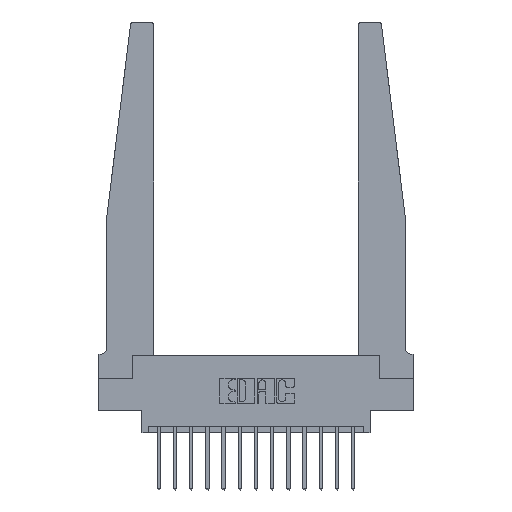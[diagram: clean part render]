
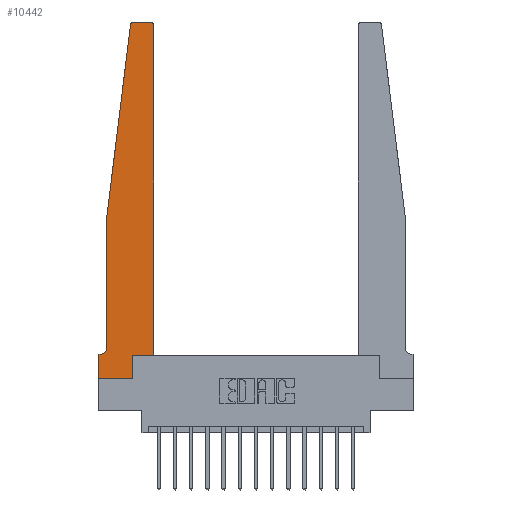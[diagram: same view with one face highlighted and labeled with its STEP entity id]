
A CAD part, top view. The second image highlights one B-rep face of the part: STEP entity #10442.
In plain terms, the highlighted planar face has unit normal (0, 0, 1).
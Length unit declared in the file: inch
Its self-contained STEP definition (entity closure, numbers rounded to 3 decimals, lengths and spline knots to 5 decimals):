
#40 = CARTESIAN_POINT ( 'NONE',  ( 0.395, 2.72, 0.37 ) ) ;
#259 = DIRECTION ( 'NONE',  ( 0., 1., 0. ) ) ;
#263 = AXIS2_PLACEMENT_3D ( 'NONE', #17476, #5307, #6751 ) ;
#320 = VECTOR ( 'NONE', #13729, 39.37008 ) ;
#450 = CARTESIAN_POINT ( 'NONE',  ( 0.015, 0.2375, 0.37 ) ) ;
#515 = LINE ( 'NONE', #7627, #7411 ) ;
#552 = EDGE_LOOP ( 'NONE', ( #8820, #11416, #11705, #750, #2528, #7859, #1773, #2253, #5050, #16981, #3275, #9507 ) ) ;
#736 = EDGE_CURVE ( 'NONE', #15306, #14373, #1399, .T. ) ;
#750 = ORIENTED_EDGE ( 'NONE', *, *, #12861, .T. ) ;
#752 = CIRCLE ( 'NONE', #17098, 0.05 ) ;
#1125 = PLANE ( 'NONE',  #3455 ) ;
#1260 = CARTESIAN_POINT ( 'NONE',  ( 0.065, 1.25, 0.37 ) ) ;
#1399 = LINE ( 'NONE', #13860, #15662 ) ;
#1417 = CARTESIAN_POINT ( 'NONE',  ( 0.2605, 0.18, 0.37 ) ) ;
#1496 = CARTESIAN_POINT ( 'NONE',  ( 0.425, 0.18, 0.37 ) ) ;
#1532 = LINE ( 'NONE', #7020, #320 ) ;
#1556 = DIRECTION ( 'NONE',  ( -1., 0., 0. ) ) ;
#1580 = CARTESIAN_POINT ( 'NONE',  ( 0., 0.1875, 0.37 ) ) ;
#1593 = VERTEX_POINT ( 'NONE', #5079 ) ;
#1635 = AXIS2_PLACEMENT_3D ( 'NONE', #40, #13786, #6817 ) ;
#1773 = ORIENTED_EDGE ( 'NONE', *, *, #5856, .T. ) ;
#1934 = VERTEX_POINT ( 'NONE', #14278 ) ;
#2253 = ORIENTED_EDGE ( 'NONE', *, *, #13636, .T. ) ;
#2420 = CARTESIAN_POINT ( 'NONE',  ( 0.2605, 0.18, 0.37 ) ) ;
#2528 = ORIENTED_EDGE ( 'NONE', *, *, #8314, .T. ) ;
#2956 = VECTOR ( 'NONE', #6786, 39.37008 ) ;
#3049 = CARTESIAN_POINT ( 'NONE',  ( 0.27653, 2.75, 0.37 ) ) ;
#3223 = DIRECTION ( 'NONE',  ( 0., -1., 0. ) ) ;
#3275 = ORIENTED_EDGE ( 'NONE', *, *, #3632, .T. ) ;
#3390 = CIRCLE ( 'NONE', #1635, 0.03 ) ;
#3455 = AXIS2_PLACEMENT_3D ( 'NONE', #9333, #15842, #5272 ) ;
#3632 = EDGE_CURVE ( 'NONE', #4372, #13907, #15254, .T. ) ;
#3851 = EDGE_CURVE ( 'NONE', #13553, #10080, #8317, .T. ) ;
#3936 = CARTESIAN_POINT ( 'NONE',  ( 0.425, 2.72, 0.37 ) ) ;
#4372 = VERTEX_POINT ( 'NONE', #1496 ) ;
#4760 = DIRECTION ( 'NONE',  ( 1., 0., 0. ) ) ;
#4801 = VERTEX_POINT ( 'NONE', #13926 ) ;
#5050 = ORIENTED_EDGE ( 'NONE', *, *, #10115, .T. ) ;
#5079 = CARTESIAN_POINT ( 'NONE',  ( 0.2605, 0., 0.37 ) ) ;
#5272 = DIRECTION ( 'NONE',  ( 1., 0., 0. ) ) ;
#5297 = CARTESIAN_POINT ( 'NONE',  ( 0.24675, 2.72367, 0.37 ) ) ;
#5307 = DIRECTION ( 'NONE',  ( 0., 0., 1. ) ) ;
#5661 = EDGE_CURVE ( 'NONE', #7172, #13553, #12382, .T. ) ;
#5856 = EDGE_CURVE ( 'NONE', #14373, #1934, #8712, .T. ) ;
#6751 = DIRECTION ( 'NONE',  ( 1., 0., 0. ) ) ;
#6786 = DIRECTION ( 'NONE',  ( -0.122, -0.992, 0. ) ) ;
#6817 = DIRECTION ( 'NONE',  ( 1., 0., 0. ) ) ;
#6829 = VERTEX_POINT ( 'NONE', #1260 ) ;
#6957 = CARTESIAN_POINT ( 'NONE',  ( 0.065, 1.25, 0.37 ) ) ;
#7020 = CARTESIAN_POINT ( 'NONE',  ( 0., 0., 0.37 ) ) ;
#7172 = VERTEX_POINT ( 'NONE', #17385 ) ;
#7411 = VECTOR ( 'NONE', #4760, 39.37008 ) ;
#7627 = CARTESIAN_POINT ( 'NONE',  ( 0.425, 0.18, 0.37 ) ) ;
#7691 = FACE_OUTER_BOUND ( 'NONE', #552, .T. ) ;
#7859 = ORIENTED_EDGE ( 'NONE', *, *, #736, .T. ) ;
#8314 = EDGE_CURVE ( 'NONE', #4801, #15306, #752, .T. ) ;
#8317 = CIRCLE ( 'NONE', #263, 0.03 ) ;
#8341 = DIRECTION ( 'NONE',  ( -1., 0., 0. ) ) ;
#8598 = LINE ( 'NONE', #10040, #16168 ) ;
#8712 = LINE ( 'NONE', #11304, #11985 ) ;
#8820 = ORIENTED_EDGE ( 'NONE', *, *, #5661, .T. ) ;
#9333 = CARTESIAN_POINT ( 'NONE',  ( 0., 0.1875, 0.37 ) ) ;
#9507 = ORIENTED_EDGE ( 'NONE', *, *, #10226, .T. ) ;
#10040 = CARTESIAN_POINT ( 'NONE',  ( 0.065, 1.25, 0.37 ) ) ;
#10051 = EDGE_CURVE ( 'NONE', #14138, #4372, #515, .T. ) ;
#10080 = VERTEX_POINT ( 'NONE', #5297 ) ;
#10115 = EDGE_CURVE ( 'NONE', #1593, #14138, #17383, .T. ) ;
#10226 = EDGE_CURVE ( 'NONE', #13907, #7172, #3390, .T. ) ;
#10307 = VECTOR ( 'NONE', #259, 39.37008 ) ;
#10442 = ADVANCED_FACE ( 'NONE', ( #7691 ), #1125, .T. ) ;
#11125 = VECTOR ( 'NONE', #13184, 39.37008 ) ;
#11304 = CARTESIAN_POINT ( 'NONE',  ( 0., 0., 0.37 ) ) ;
#11416 = ORIENTED_EDGE ( 'NONE', *, *, #3851, .T. ) ;
#11705 = ORIENTED_EDGE ( 'NONE', *, *, #17003, .T. ) ;
#11985 = VECTOR ( 'NONE', #3223, 39.37008 ) ;
#12186 = DIRECTION ( 'NONE',  ( -1., 0., 0. ) ) ;
#12215 = CARTESIAN_POINT ( 'NONE',  ( 0.25, 2.75, 0.37 ) ) ;
#12382 = LINE ( 'NONE', #12215, #16842 ) ;
#12579 = CARTESIAN_POINT ( 'NONE',  ( 0.425, 0.18, 0.37 ) ) ;
#12589 = DIRECTION ( 'NONE',  ( 0., 0., -1. ) ) ;
#12861 = EDGE_CURVE ( 'NONE', #6829, #4801, #8598, .T. ) ;
#13184 = DIRECTION ( 'NONE',  ( 0., 1., 0. ) ) ;
#13553 = VERTEX_POINT ( 'NONE', #3049 ) ;
#13636 = EDGE_CURVE ( 'NONE', #1934, #1593, #1532, .T. ) ;
#13729 = DIRECTION ( 'NONE',  ( 1., 0., 0. ) ) ;
#13786 = DIRECTION ( 'NONE',  ( 0., 0., 1. ) ) ;
#13860 = CARTESIAN_POINT ( 'NONE',  ( 0.065, 0.1875, 0.37 ) ) ;
#13907 = VERTEX_POINT ( 'NONE', #3936 ) ;
#13926 = CARTESIAN_POINT ( 'NONE',  ( 0.065, 0.2375, 0.37 ) ) ;
#14138 = VERTEX_POINT ( 'NONE', #1417 ) ;
#14278 = CARTESIAN_POINT ( 'NONE',  ( 0., 0., 0.37 ) ) ;
#14373 = VERTEX_POINT ( 'NONE', #1580 ) ;
#15097 = LINE ( 'NONE', #6957, #2956 ) ;
#15228 = CARTESIAN_POINT ( 'NONE',  ( 0.015, 0.1875, 0.37 ) ) ;
#15254 = LINE ( 'NONE', #12579, #10307 ) ;
#15306 = VERTEX_POINT ( 'NONE', #15228 ) ;
#15662 = VECTOR ( 'NONE', #12186, 39.37008 ) ;
#15666 = DIRECTION ( 'NONE',  ( 0., -1., 0. ) ) ;
#15842 = DIRECTION ( 'NONE',  ( 0., 0., 1. ) ) ;
#16168 = VECTOR ( 'NONE', #15666, 39.37008 ) ;
#16842 = VECTOR ( 'NONE', #8341, 39.37008 ) ;
#16981 = ORIENTED_EDGE ( 'NONE', *, *, #10051, .T. ) ;
#17003 = EDGE_CURVE ( 'NONE', #10080, #6829, #15097, .T. ) ;
#17098 = AXIS2_PLACEMENT_3D ( 'NONE', #450, #12589, #1556 ) ;
#17383 = LINE ( 'NONE', #2420, #11125 ) ;
#17385 = CARTESIAN_POINT ( 'NONE',  ( 0.395, 2.75, 0.37 ) ) ;
#17476 = CARTESIAN_POINT ( 'NONE',  ( 0.27653, 2.72, 0.37 ) ) ;
